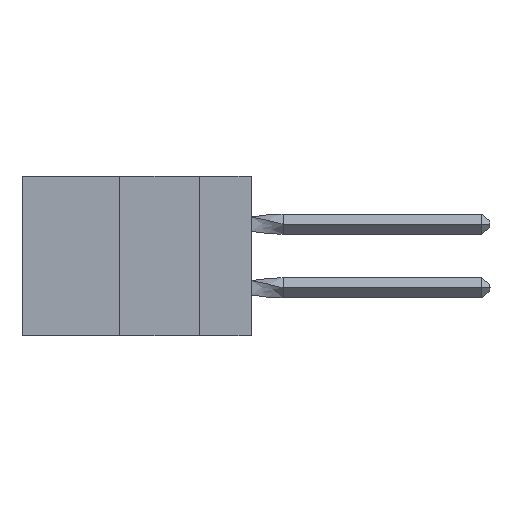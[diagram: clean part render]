
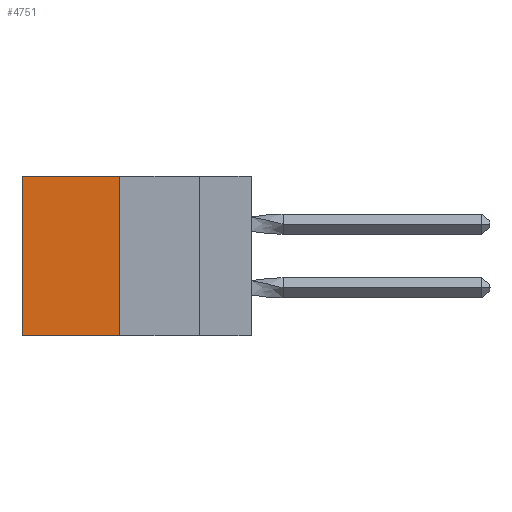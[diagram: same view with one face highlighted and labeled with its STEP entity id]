
A CAD part, left-side view. The second image highlights one B-rep face of the part: STEP entity #4751.
In plain terms, the highlighted planar face has unit normal (-1, 0, 0).
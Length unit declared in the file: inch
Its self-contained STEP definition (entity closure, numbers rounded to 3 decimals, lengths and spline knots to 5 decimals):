
#284 = EDGE_LOOP ( 'NONE', ( #15461, #10019, #4892, #2924 ) ) ;
#1513 = VERTEX_POINT ( 'NONE', #10520 ) ;
#1927 = CARTESIAN_POINT ( 'NONE',  ( 0.305, 0.72, -0.5 ) ) ;
#2530 = CARTESIAN_POINT ( 'NONE',  ( 0.305, 0.72, -0.5 ) ) ;
#2924 = ORIENTED_EDGE ( 'NONE', *, *, #6030, .T. ) ;
#3928 = DIRECTION ( 'NONE',  ( 0., 0., -1. ) ) ;
#4751 = ADVANCED_FACE ( 'NONE', ( #17268 ), #12678, .F. ) ;
#4892 = ORIENTED_EDGE ( 'NONE', *, *, #17413, .F. ) ;
#5960 = CARTESIAN_POINT ( 'NONE',  ( 0.305, 0.413, -0.5 ) ) ;
#6030 = EDGE_CURVE ( 'NONE', #16847, #1513, #7622, .T. ) ;
#7006 = DIRECTION ( 'NONE',  ( 0., 1., 0. ) ) ;
#7451 = DIRECTION ( 'NONE',  ( 0., 0., -1. ) ) ;
#7622 = LINE ( 'NONE', #8613, #21337 ) ;
#7741 = CARTESIAN_POINT ( 'NONE',  ( 0.305, 0.413, -0.5 ) ) ;
#8613 = CARTESIAN_POINT ( 'NONE',  ( 0.305, 0.413, 0. ) ) ;
#9163 = EDGE_CURVE ( 'NONE', #20603, #13216, #16546, .T. ) ;
#10019 = ORIENTED_EDGE ( 'NONE', *, *, #9163, .F. ) ;
#10520 = CARTESIAN_POINT ( 'NONE',  ( 0.305, 0.72, 0. ) ) ;
#10599 = LINE ( 'NONE', #2530, #13157 ) ;
#10651 = AXIS2_PLACEMENT_3D ( 'NONE', #15855, #15727, #7451 ) ;
#11136 = VECTOR ( 'NONE', #7006, 39.37008 ) ;
#12678 = PLANE ( 'NONE',  #10651 ) ;
#13157 = VECTOR ( 'NONE', #3928, 39.37008 ) ;
#13216 = VERTEX_POINT ( 'NONE', #1927 ) ;
#13593 = DIRECTION ( 'NONE',  ( 0., 1., 0. ) ) ;
#14190 = CARTESIAN_POINT ( 'NONE',  ( 0.305, 0.413, 0. ) ) ;
#15428 = CARTESIAN_POINT ( 'NONE',  ( 0.305, 0.413, -0.5 ) ) ;
#15461 = ORIENTED_EDGE ( 'NONE', *, *, #17858, .T. ) ;
#15530 = VECTOR ( 'NONE', #19342, 39.37008 ) ;
#15727 = DIRECTION ( 'NONE',  ( 1., 0., 0. ) ) ;
#15855 = CARTESIAN_POINT ( 'NONE',  ( 0.305, 0.413, -0.5 ) ) ;
#16546 = LINE ( 'NONE', #15428, #11136 ) ;
#16847 = VERTEX_POINT ( 'NONE', #14190 ) ;
#17268 = FACE_OUTER_BOUND ( 'NONE', #284, .T. ) ;
#17413 = EDGE_CURVE ( 'NONE', #16847, #20603, #19646, .T. ) ;
#17858 = EDGE_CURVE ( 'NONE', #1513, #13216, #10599, .T. ) ;
#19342 = DIRECTION ( 'NONE',  ( 0., 0., -1. ) ) ;
#19646 = LINE ( 'NONE', #7741, #15530 ) ;
#20603 = VERTEX_POINT ( 'NONE', #5960 ) ;
#21337 = VECTOR ( 'NONE', #13593, 39.37008 ) ;
